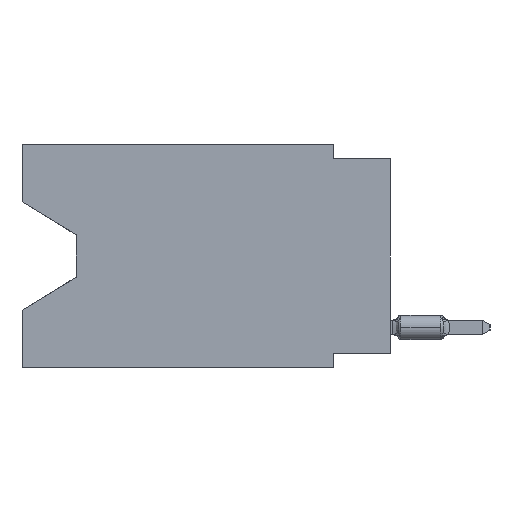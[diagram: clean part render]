
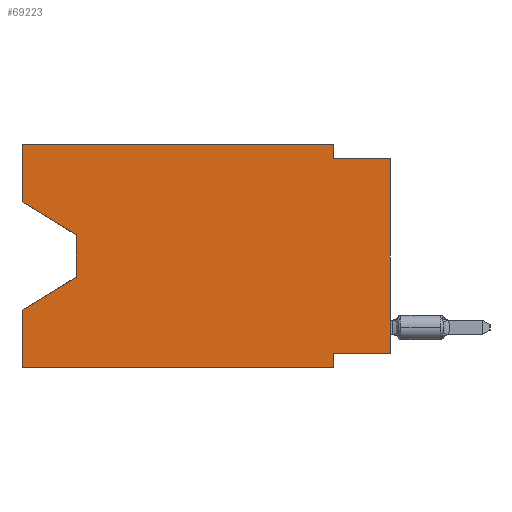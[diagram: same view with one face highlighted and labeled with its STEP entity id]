
A CAD part, left-side view. The second image highlights one B-rep face of the part: STEP entity #69223.
In plain terms, the highlighted planar face has unit normal (-1, 0, 0).
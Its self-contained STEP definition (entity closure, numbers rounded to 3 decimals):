
#484 = VERTEX_POINT ( 'NONE', #40932 ) ;
#1421 = VECTOR ( 'NONE', #32665, 1000. ) ;
#3665 = ORIENTED_EDGE ( 'NONE', *, *, #55319, .F. ) ;
#4044 = DIRECTION ( 'NONE',  ( 0., 0., -1. ) ) ;
#4762 = CARTESIAN_POINT ( 'NONE',  ( 0., 13.97, -5.893 ) ) ;
#6357 = VERTEX_POINT ( 'NONE', #37913 ) ;
#6595 = CARTESIAN_POINT ( 'NONE',  ( 0., 0., -0.635 ) ) ;
#7037 = LINE ( 'NONE', #44821, #44393 ) ;
#7412 = ORIENTED_EDGE ( 'NONE', *, *, #20343, .T. ) ;
#8006 = DIRECTION ( 'NONE',  ( 0., 0.855, -0.519 ) ) ;
#8432 = LINE ( 'NONE', #76674, #1421 ) ;
#8995 = LINE ( 'NONE', #22941, #40450 ) ;
#10696 = DIRECTION ( 'NONE',  ( 0., 0., 1. ) ) ;
#11673 = ORIENTED_EDGE ( 'NONE', *, *, #62949, .T. ) ;
#12923 = VERTEX_POINT ( 'NONE', #59742 ) ;
#13502 = EDGE_CURVE ( 'NONE', #27814, #58659, #47113, .T. ) ;
#13590 = DIRECTION ( 'NONE',  ( 0., 0., 1. ) ) ;
#14742 = VECTOR ( 'NONE', #61694, 1000. ) ;
#16734 = VECTOR ( 'NONE', #57539, 1000. ) ;
#16872 = LINE ( 'NONE', #66990, #20114 ) ;
#17238 = EDGE_CURVE ( 'NONE', #56369, #69142, #54461, .T. ) ;
#17508 = ORIENTED_EDGE ( 'NONE', *, *, #63986, .F. ) ;
#18447 = VECTOR ( 'NONE', #52074, 1000. ) ;
#18925 = CARTESIAN_POINT ( 'NONE',  ( 0., 13.97, -4.013 ) ) ;
#19110 = VERTEX_POINT ( 'NONE', #79550 ) ;
#19938 = AXIS2_PLACEMENT_3D ( 'NONE', #58762, #47643, #52587 ) ;
#20114 = VECTOR ( 'NONE', #10696, 1000. ) ;
#20343 = EDGE_CURVE ( 'NONE', #77363, #65994, #30219, .T. ) ;
#22941 = CARTESIAN_POINT ( 'NONE',  ( 0., 2.54, 0. ) ) ;
#23228 = DIRECTION ( 'NONE',  ( 0., -0.855, -0.519 ) ) ;
#27061 = CARTESIAN_POINT ( 'NONE',  ( 0., 16.383, 0. ) ) ;
#27638 = ORIENTED_EDGE ( 'NONE', *, *, #53440, .T. ) ;
#27814 = VERTEX_POINT ( 'NONE', #27061 ) ;
#27939 = FACE_OUTER_BOUND ( 'NONE', #50837, .T. ) ;
#28885 = VERTEX_POINT ( 'NONE', #69004 ) ;
#29580 = CARTESIAN_POINT ( 'NONE',  ( 0., 16.383, -2.546 ) ) ;
#30219 = LINE ( 'NONE', #74207, #78750 ) ;
#30690 = DIRECTION ( 'NONE',  ( 0., 0., 1. ) ) ;
#31093 = LINE ( 'NONE', #38498, #52669 ) ;
#31271 = CARTESIAN_POINT ( 'NONE',  ( 0., 2.54, -9.906 ) ) ;
#32665 = DIRECTION ( 'NONE',  ( 0., 1., 0. ) ) ;
#32848 = LINE ( 'NONE', #6595, #16734 ) ;
#34466 = ORIENTED_EDGE ( 'NONE', *, *, #60754, .T. ) ;
#37913 = CARTESIAN_POINT ( 'NONE',  ( 0., 2.54, -9.271 ) ) ;
#38498 = CARTESIAN_POINT ( 'NONE',  ( 0., 16.383, 0. ) ) ;
#40450 = VECTOR ( 'NONE', #4044, 1000. ) ;
#40656 = PLANE ( 'NONE',  #19938 ) ;
#40932 = CARTESIAN_POINT ( 'NONE',  ( 0., 16.383, -9.906 ) ) ;
#41655 = LINE ( 'NONE', #18925, #79800 ) ;
#42141 = CARTESIAN_POINT ( 'NONE',  ( 0., 16.383, -2.546 ) ) ;
#43619 = CARTESIAN_POINT ( 'NONE',  ( 0., 16.383, -9.906 ) ) ;
#44051 = ORIENTED_EDGE ( 'NONE', *, *, #13502, .F. ) ;
#44393 = VECTOR ( 'NONE', #13590, 1000. ) ;
#44600 = LINE ( 'NONE', #64290, #61487 ) ;
#44821 = CARTESIAN_POINT ( 'NONE',  ( 0., 0., 0. ) ) ;
#45789 = ORIENTED_EDGE ( 'NONE', *, *, #17238, .T. ) ;
#47113 = LINE ( 'NONE', #59043, #18447 ) ;
#47643 = DIRECTION ( 'NONE',  ( 1., 0., 0. ) ) ;
#49365 = LINE ( 'NONE', #43619, #14742 ) ;
#50837 = EDGE_LOOP ( 'NONE', ( #45789, #11673, #7412, #80973, #34466, #17508, #65457, #27638, #55949, #78272, #44051, #3665 ) ) ;
#52074 = DIRECTION ( 'NONE',  ( 0., -1., 0. ) ) ;
#52587 = DIRECTION ( 'NONE',  ( 0., 0., -1. ) ) ;
#52669 = VECTOR ( 'NONE', #30690, 1000. ) ;
#53017 = CARTESIAN_POINT ( 'NONE',  ( 0., 16.383, -7.36 ) ) ;
#53440 = EDGE_CURVE ( 'NONE', #19110, #12923, #7037, .T. ) ;
#54366 = VECTOR ( 'NONE', #23228, 1000. ) ;
#54461 = LINE ( 'NONE', #42141, #54366 ) ;
#55319 = EDGE_CURVE ( 'NONE', #56369, #27814, #31093, .T. ) ;
#55949 = ORIENTED_EDGE ( 'NONE', *, *, #77942, .F. ) ;
#56369 = VERTEX_POINT ( 'NONE', #29580 ) ;
#56731 = DIRECTION ( 'NONE',  ( 0., 0., -1. ) ) ;
#57539 = DIRECTION ( 'NONE',  ( 0., -1., 0. ) ) ;
#58659 = VERTEX_POINT ( 'NONE', #62706 ) ;
#58762 = CARTESIAN_POINT ( 'NONE',  ( 0., 16.383, 0. ) ) ;
#58874 = EDGE_CURVE ( 'NONE', #19110, #6357, #8432, .T. ) ;
#59043 = CARTESIAN_POINT ( 'NONE',  ( 0., 16.383, 0. ) ) ;
#59742 = CARTESIAN_POINT ( 'NONE',  ( 0., 0., -0.635 ) ) ;
#60754 = EDGE_CURVE ( 'NONE', #484, #60771, #49365, .T. ) ;
#60771 = VERTEX_POINT ( 'NONE', #31271 ) ;
#61487 = VECTOR ( 'NONE', #69658, 1000. ) ;
#61694 = DIRECTION ( 'NONE',  ( 0., -1., 0. ) ) ;
#62706 = CARTESIAN_POINT ( 'NONE',  ( 0., 2.54, 0. ) ) ;
#62949 = EDGE_CURVE ( 'NONE', #69142, #77363, #41655, .T. ) ;
#63986 = EDGE_CURVE ( 'NONE', #6357, #60771, #44600, .T. ) ;
#64290 = CARTESIAN_POINT ( 'NONE',  ( 0., 2.54, -9.906 ) ) ;
#65457 = ORIENTED_EDGE ( 'NONE', *, *, #58874, .F. ) ;
#65994 = VERTEX_POINT ( 'NONE', #53017 ) ;
#66990 = CARTESIAN_POINT ( 'NONE',  ( 0., 16.383, 0. ) ) ;
#69004 = CARTESIAN_POINT ( 'NONE',  ( 0., 2.54, -0.635 ) ) ;
#69142 = VERTEX_POINT ( 'NONE', #77679 ) ;
#69223 = ADVANCED_FACE ( 'NONE', ( #27939 ), #40656, .F. ) ;
#69658 = DIRECTION ( 'NONE',  ( 0., 0., -1. ) ) ;
#71339 = EDGE_CURVE ( 'NONE', #484, #65994, #16872, .T. ) ;
#74207 = CARTESIAN_POINT ( 'NONE',  ( 0., 13.97, -5.893 ) ) ;
#76674 = CARTESIAN_POINT ( 'NONE',  ( 0., 0., -9.271 ) ) ;
#77363 = VERTEX_POINT ( 'NONE', #4762 ) ;
#77679 = CARTESIAN_POINT ( 'NONE',  ( 0., 13.97, -4.013 ) ) ;
#77942 = EDGE_CURVE ( 'NONE', #28885, #12923, #32848, .T. ) ;
#78272 = ORIENTED_EDGE ( 'NONE', *, *, #78649, .F. ) ;
#78649 = EDGE_CURVE ( 'NONE', #58659, #28885, #8995, .T. ) ;
#78750 = VECTOR ( 'NONE', #8006, 1000. ) ;
#79550 = CARTESIAN_POINT ( 'NONE',  ( 0., 0., -9.271 ) ) ;
#79800 = VECTOR ( 'NONE', #56731, 1000. ) ;
#80973 = ORIENTED_EDGE ( 'NONE', *, *, #71339, .F. ) ;
